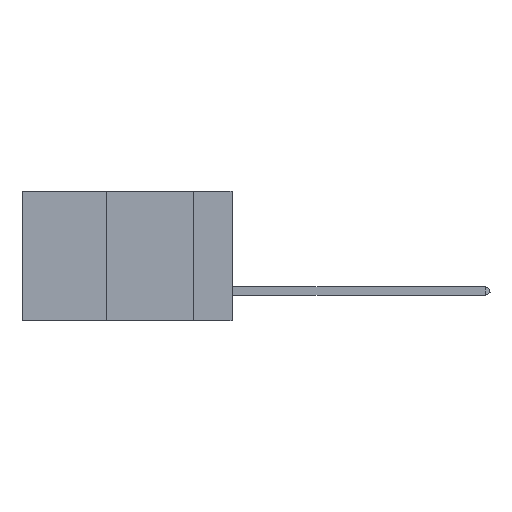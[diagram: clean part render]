
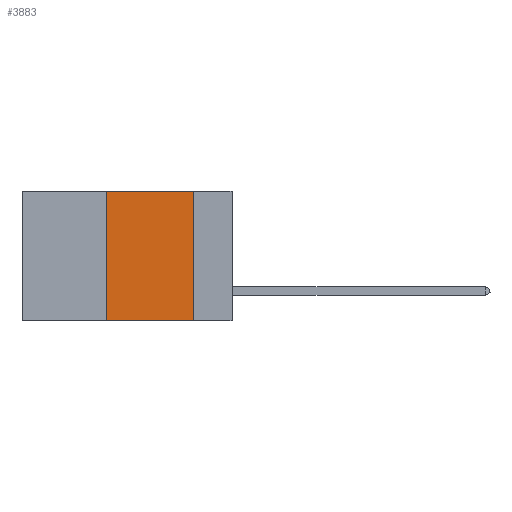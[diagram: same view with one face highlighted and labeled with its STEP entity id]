
A CAD part, left-side view. The second image highlights one B-rep face of the part: STEP entity #3883.
In plain terms, the highlighted planar face has unit normal (-1, 0, 0).
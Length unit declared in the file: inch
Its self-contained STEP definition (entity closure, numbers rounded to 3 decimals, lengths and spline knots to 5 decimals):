
#384 = LINE ( 'NONE', #18271, #17933 ) ;
#2397 = EDGE_CURVE ( 'NONE', #16374, #13482, #384, .T. ) ;
#3613 = EDGE_CURVE ( 'NONE', #10272, #16374, #15334, .T. ) ;
#3883 = ADVANCED_FACE ( 'NONE', ( #11743 ), #22162, .F. ) ;
#4173 = LINE ( 'NONE', #17038, #29851 ) ;
#6780 = DIRECTION ( 'NONE',  ( 0., 0., 1. ) ) ;
#7751 = ORIENTED_EDGE ( 'NONE', *, *, #22540, .F. ) ;
#8018 = VECTOR ( 'NONE', #27908, 39.37008 ) ;
#10272 = VERTEX_POINT ( 'NONE', #13938 ) ;
#11743 = FACE_OUTER_BOUND ( 'NONE', #20091, .T. ) ;
#12056 = DIRECTION ( 'NONE',  ( 1., 0., 0. ) ) ;
#13482 = VERTEX_POINT ( 'NONE', #15817 ) ;
#13938 = CARTESIAN_POINT ( 'NONE',  ( 0., 0.36, 0. ) ) ;
#15334 = LINE ( 'NONE', #22994, #8018 ) ;
#15817 = CARTESIAN_POINT ( 'NONE',  ( 0., 0.11, -0.37 ) ) ;
#16374 = VERTEX_POINT ( 'NONE', #19694 ) ;
#17038 = CARTESIAN_POINT ( 'NONE',  ( 0., 0.36, 0. ) ) ;
#17933 = VECTOR ( 'NONE', #28240, 39.37008 ) ;
#18271 = CARTESIAN_POINT ( 'NONE',  ( 0., 0.11, 0. ) ) ;
#19154 = CARTESIAN_POINT ( 'NONE',  ( 0., 0.6, -0.37 ) ) ;
#19694 = CARTESIAN_POINT ( 'NONE',  ( 0., 0.11, 0. ) ) ;
#20091 = EDGE_LOOP ( 'NONE', ( #30509, #20092, #7751, #26643 ) ) ;
#20092 = ORIENTED_EDGE ( 'NONE', *, *, #3613, .F. ) ;
#21505 = AXIS2_PLACEMENT_3D ( 'NONE', #24441, #12056, #21688 ) ;
#21559 = VECTOR ( 'NONE', #29107, 39.37008 ) ;
#21688 = DIRECTION ( 'NONE',  ( 0., 0., -1. ) ) ;
#22162 = PLANE ( 'NONE',  #21505 ) ;
#22540 = EDGE_CURVE ( 'NONE', #23102, #10272, #4173, .T. ) ;
#22617 = EDGE_CURVE ( 'NONE', #23102, #13482, #31552, .T. ) ;
#22994 = CARTESIAN_POINT ( 'NONE',  ( 0., 0.6, 0. ) ) ;
#23102 = VERTEX_POINT ( 'NONE', #24769 ) ;
#24441 = CARTESIAN_POINT ( 'NONE',  ( 0., 0.6, 0. ) ) ;
#24769 = CARTESIAN_POINT ( 'NONE',  ( 0., 0.36, -0.37 ) ) ;
#26643 = ORIENTED_EDGE ( 'NONE', *, *, #22617, .T. ) ;
#27908 = DIRECTION ( 'NONE',  ( 0., -1., 0. ) ) ;
#28240 = DIRECTION ( 'NONE',  ( 0., 0., -1. ) ) ;
#29107 = DIRECTION ( 'NONE',  ( 0., -1., 0. ) ) ;
#29851 = VECTOR ( 'NONE', #6780, 39.37008 ) ;
#30509 = ORIENTED_EDGE ( 'NONE', *, *, #2397, .F. ) ;
#31552 = LINE ( 'NONE', #19154, #21559 ) ;
